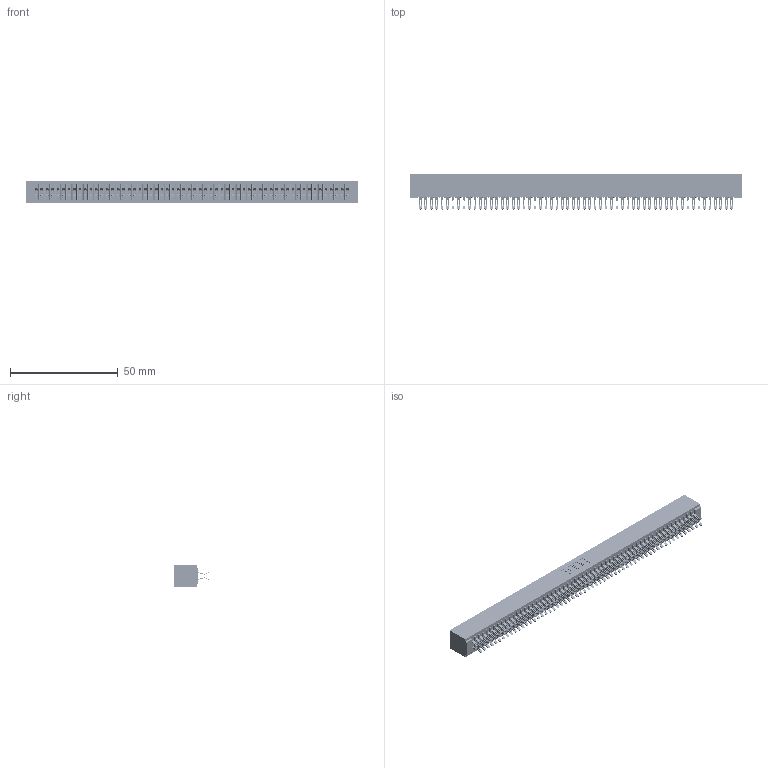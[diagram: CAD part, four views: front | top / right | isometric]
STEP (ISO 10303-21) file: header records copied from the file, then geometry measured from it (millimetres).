
FILE_DESCRIPTION (( 'STEP AP203' ), '1' );
FILE_NAME ('341-116-555-201.STEP', '2018-08-08T14:03:38', ( '' ), ( '' ), 'SwSTEP 2.0', 'SolidWorks 2016', '' );
FILE_SCHEMA (( 'CONFIG_CONTROL_DESIGN' ));
Length unit declared in the file: inch
Products named in the file (3): 341 Part_No Mounting Lugs; 341-292-001_341-292-155; 341-116-555-201
Assembly tree (117 placements, depth 2):
  341-116-555-201
    341 Part_No Mounting Lugs
    341-292-001_341-292-155  x116
Bounding box: 154.31 x 16.31 x 10.16 mm (x, y, z)
Volume: 11792.1 mm3; surface area: 23046.4 mm2
Topology: 117 solids, 117 shells, 9156 faces, 27378 edges, 17822 vertices
Faces by surface type: plane 4936, cylinder 3988, sphere 118, torus 114
Entity records: 68253 total; most frequent: CARTESIAN_POINT 11360, ORIENTED_EDGE 11280, DIRECTION 11002, EDGE_CURVE 5640, VECTOR 4562, LINE 4562, VERTEX_POINT 3562, AXIS2_PLACEMENT_3D 3220
